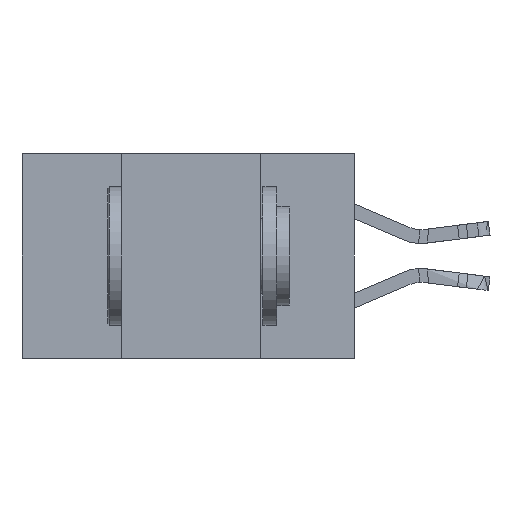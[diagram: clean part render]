
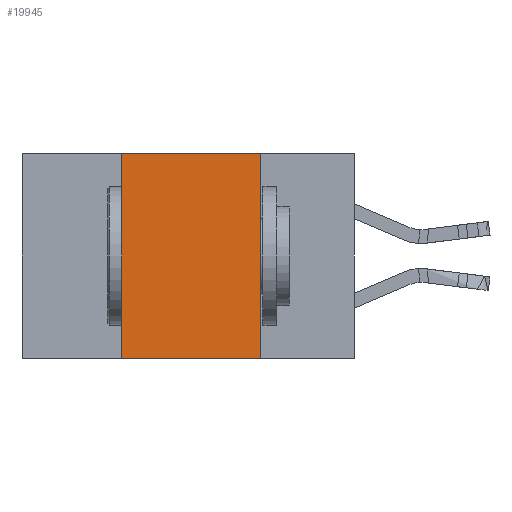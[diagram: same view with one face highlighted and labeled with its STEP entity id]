
A CAD part, left-side view. The second image highlights one B-rep face of the part: STEP entity #19945.
In plain terms, the highlighted planar face has unit normal (-1, 0, 0).
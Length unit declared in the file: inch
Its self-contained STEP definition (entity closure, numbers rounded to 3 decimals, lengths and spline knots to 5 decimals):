
#2129 = PLANE ( 'NONE',  #4283 ) ;
#4283 = AXIS2_PLACEMENT_3D ( 'NONE', #15613, #17505, #28556 ) ;
#4630 = VERTEX_POINT ( 'NONE', #7893 ) ;
#5095 = DIRECTION ( 'NONE',  ( 0., 0., -1. ) ) ;
#5868 = ORIENTED_EDGE ( 'NONE', *, *, #11362, .T. ) ;
#6650 = FACE_OUTER_BOUND ( 'NONE', #8121, .T. ) ;
#7613 = CARTESIAN_POINT ( 'NONE',  ( 0., 0.42, 0. ) ) ;
#7893 = CARTESIAN_POINT ( 'NONE',  ( 0., 0.42, -0.37 ) ) ;
#8121 = EDGE_LOOP ( 'NONE', ( #18004, #20554, #28402, #5868 ) ) ;
#9117 = VECTOR ( 'NONE', #5095, 39.37008 ) ;
#9155 = VECTOR ( 'NONE', #16002, 39.37008 ) ;
#9715 = CARTESIAN_POINT ( 'NONE',  ( 0., 0.17, -0.37 ) ) ;
#10037 = CARTESIAN_POINT ( 'NONE',  ( 0., 0.6, 0. ) ) ;
#10981 = VECTOR ( 'NONE', #16999, 39.37008 ) ;
#11362 = EDGE_CURVE ( 'NONE', #4630, #15894, #14666, .T. ) ;
#11530 = EDGE_CURVE ( 'NONE', #11601, #15894, #16101, .T. ) ;
#11601 = VERTEX_POINT ( 'NONE', #18162 ) ;
#11804 = LINE ( 'NONE', #10037, #9155 ) ;
#12507 = CARTESIAN_POINT ( 'NONE',  ( 0., 0.6, -0.37 ) ) ;
#12563 = EDGE_CURVE ( 'NONE', #22009, #11601, #11804, .T. ) ;
#13792 = VECTOR ( 'NONE', #19410, 39.37008 ) ;
#14340 = CARTESIAN_POINT ( 'NONE',  ( 0., 0.17, -0.37 ) ) ;
#14666 = LINE ( 'NONE', #12507, #10981 ) ;
#15613 = CARTESIAN_POINT ( 'NONE',  ( 0., 0.6, 0. ) ) ;
#15894 = VERTEX_POINT ( 'NONE', #14340 ) ;
#16002 = DIRECTION ( 'NONE',  ( 0., -1., 0. ) ) ;
#16101 = LINE ( 'NONE', #9715, #9117 ) ;
#16999 = DIRECTION ( 'NONE',  ( 0., -1., 0. ) ) ;
#17225 = LINE ( 'NONE', #22030, #13792 ) ;
#17505 = DIRECTION ( 'NONE',  ( 1., 0., 0. ) ) ;
#18004 = ORIENTED_EDGE ( 'NONE', *, *, #11530, .F. ) ;
#18162 = CARTESIAN_POINT ( 'NONE',  ( 0., 0.17, 0. ) ) ;
#19410 = DIRECTION ( 'NONE',  ( 0., 0., 1. ) ) ;
#19945 = ADVANCED_FACE ( 'NONE', ( #6650 ), #2129, .F. ) ;
#20554 = ORIENTED_EDGE ( 'NONE', *, *, #12563, .F. ) ;
#22009 = VERTEX_POINT ( 'NONE', #7613 ) ;
#22030 = CARTESIAN_POINT ( 'NONE',  ( 0., 0.42, -0.37 ) ) ;
#26452 = EDGE_CURVE ( 'NONE', #4630, #22009, #17225, .T. ) ;
#28402 = ORIENTED_EDGE ( 'NONE', *, *, #26452, .F. ) ;
#28556 = DIRECTION ( 'NONE',  ( 0., 0., -1. ) ) ;
